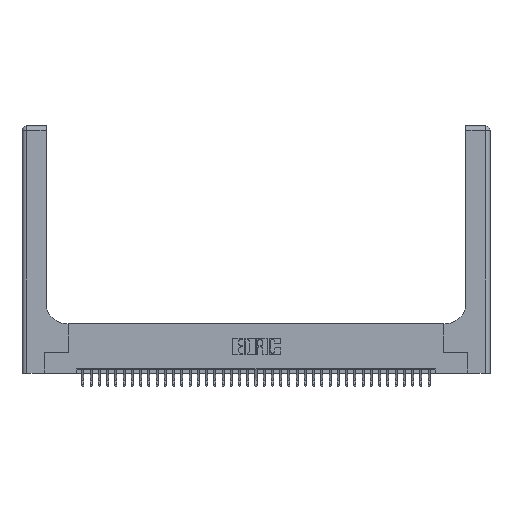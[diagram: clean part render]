
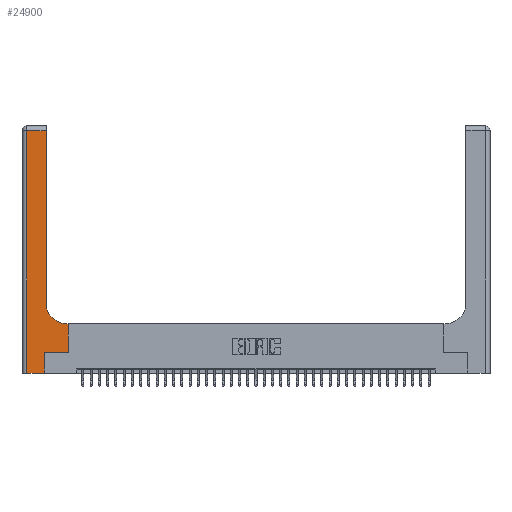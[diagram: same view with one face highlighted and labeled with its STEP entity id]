
A CAD part, top view. The second image highlights one B-rep face of the part: STEP entity #24900.
In plain terms, the highlighted planar face has unit normal (0, 0, 1).
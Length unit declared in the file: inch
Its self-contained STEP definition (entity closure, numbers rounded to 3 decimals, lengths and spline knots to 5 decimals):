
#95 = DIRECTION ( 'NONE',  ( 1., 0., 0. ) ) ;
#449 = VECTOR ( 'NONE', #18951, 39.37008 ) ;
#495 = EDGE_CURVE ( 'NONE', #4939, #36601, #34868, .T. ) ;
#773 = CARTESIAN_POINT ( 'NONE',  ( 0.2915, 0.6, 0.37 ) ) ;
#952 = LINE ( 'NONE', #773, #449 ) ;
#2243 = CARTESIAN_POINT ( 'NONE',  ( 0.5415, 0.6, 0.37 ) ) ;
#2503 = CARTESIAN_POINT ( 'NONE',  ( 0.06, 3., 0.37 ) ) ;
#2934 = VERTEX_POINT ( 'NONE', #2243 ) ;
#3071 = CARTESIAN_POINT ( 'NONE',  ( 0.5585, 0.25, 0.37 ) ) ;
#3129 = ORIENTED_EDGE ( 'NONE', *, *, #9283, .T. ) ;
#3180 = LINE ( 'NONE', #18246, #21992 ) ;
#4939 = VERTEX_POINT ( 'NONE', #29171 ) ;
#6209 = CARTESIAN_POINT ( 'NONE',  ( 0.06, 2.94, 0.37 ) ) ;
#6495 = ORIENTED_EDGE ( 'NONE', *, *, #19314, .T. ) ;
#7766 = DIRECTION ( 'NONE',  ( -1., 0., 0. ) ) ;
#8677 = PLANE ( 'NONE',  #22682 ) ;
#8778 = CARTESIAN_POINT ( 'NONE',  ( 0., 0., 0.37 ) ) ;
#9073 = ORIENTED_EDGE ( 'NONE', *, *, #16976, .T. ) ;
#9089 = CARTESIAN_POINT ( 'NONE',  ( 0., 3., 0.37 ) ) ;
#9207 = DIRECTION ( 'NONE',  ( 0., 1., 0. ) ) ;
#9229 = CARTESIAN_POINT ( 'NONE',  ( 0.06, 0., 0.37 ) ) ;
#9283 = EDGE_CURVE ( 'NONE', #36601, #21958, #17452, .T. ) ;
#9290 = EDGE_CURVE ( 'NONE', #37697, #36356, #27822, .T. ) ;
#9387 = LINE ( 'NONE', #2503, #24444 ) ;
#11012 = CARTESIAN_POINT ( 'NONE',  ( 0.5585, 0.25, 0.37 ) ) ;
#11868 = VECTOR ( 'NONE', #32856, 39.37008 ) ;
#12424 = ORIENTED_EDGE ( 'NONE', *, *, #9290, .T. ) ;
#13799 = CARTESIAN_POINT ( 'NONE',  ( 0., 2.94, 0.37 ) ) ;
#14481 = ORIENTED_EDGE ( 'NONE', *, *, #15938, .T. ) ;
#14742 = CARTESIAN_POINT ( 'NONE',  ( 0.5415, 0.85, 0.37 ) ) ;
#15938 = EDGE_CURVE ( 'NONE', #21958, #2934, #952, .T. ) ;
#16024 = VERTEX_POINT ( 'NONE', #6209 ) ;
#16976 = EDGE_CURVE ( 'NONE', #35573, #31599, #29206, .T. ) ;
#17452 = LINE ( 'NONE', #3071, #19821 ) ;
#17720 = CARTESIAN_POINT ( 'NONE',  ( 0.5585, 0.6, 0.37 ) ) ;
#18168 = VECTOR ( 'NONE', #7766, 39.37008 ) ;
#18206 = DIRECTION ( 'NONE',  ( 0., 1., 0. ) ) ;
#18246 = CARTESIAN_POINT ( 'NONE',  ( 0.269, 0., 0.37 ) ) ;
#18400 = DIRECTION ( 'NONE',  ( 1., 0., 0. ) ) ;
#18951 = DIRECTION ( 'NONE',  ( -1., 0., 0. ) ) ;
#19314 = EDGE_CURVE ( 'NONE', #31599, #16024, #34228, .T. ) ;
#19821 = VECTOR ( 'NONE', #18206, 39.37008 ) ;
#21958 = VERTEX_POINT ( 'NONE', #17720 ) ;
#21992 = VECTOR ( 'NONE', #9207, 39.37008 ) ;
#22091 = EDGE_CURVE ( 'NONE', #36356, #4939, #3180, .T. ) ;
#22132 = DIRECTION ( 'NONE',  ( 0., 1., 0. ) ) ;
#22682 = AXIS2_PLACEMENT_3D ( 'NONE', #9089, #29572, #32757 ) ;
#24063 = VECTOR ( 'NONE', #22132, 39.37008 ) ;
#24444 = VECTOR ( 'NONE', #34088, 39.37008 ) ;
#24900 = ADVANCED_FACE ( 'NONE', ( #31172 ), #8677, .F. ) ;
#25110 = ORIENTED_EDGE ( 'NONE', *, *, #35725, .T. ) ;
#26713 = DIRECTION ( 'NONE',  ( 0., 0., -1. ) ) ;
#27822 = LINE ( 'NONE', #8778, #11868 ) ;
#29027 = ORIENTED_EDGE ( 'NONE', *, *, #495, .T. ) ;
#29171 = CARTESIAN_POINT ( 'NONE',  ( 0.269, 0.25, 0.37 ) ) ;
#29206 = LINE ( 'NONE', #37038, #24063 ) ;
#29541 = CIRCLE ( 'NONE', #37992, 0.25 ) ;
#29572 = DIRECTION ( 'NONE',  ( 0., 0., -1. ) ) ;
#30585 = EDGE_LOOP ( 'NONE', ( #9073, #6495, #25110, #12424, #35002, #29027, #3129, #14481, #30800 ) ) ;
#30800 = ORIENTED_EDGE ( 'NONE', *, *, #36248, .T. ) ;
#31172 = FACE_OUTER_BOUND ( 'NONE', #30585, .T. ) ;
#31599 = VERTEX_POINT ( 'NONE', #34685 ) ;
#31879 = CARTESIAN_POINT ( 'NONE',  ( 0.2915, 0.85, 0.37 ) ) ;
#32757 = DIRECTION ( 'NONE',  ( -1., 0., 0. ) ) ;
#32856 = DIRECTION ( 'NONE',  ( 1., 0., 0. ) ) ;
#33786 = CARTESIAN_POINT ( 'NONE',  ( 0.269, 0., 0.37 ) ) ;
#34088 = DIRECTION ( 'NONE',  ( 0., -1., 0. ) ) ;
#34228 = LINE ( 'NONE', #13799, #18168 ) ;
#34685 = CARTESIAN_POINT ( 'NONE',  ( 0.2915, 2.94, 0.37 ) ) ;
#34868 = LINE ( 'NONE', #38985, #35339 ) ;
#35002 = ORIENTED_EDGE ( 'NONE', *, *, #22091, .T. ) ;
#35339 = VECTOR ( 'NONE', #18400, 39.37008 ) ;
#35573 = VERTEX_POINT ( 'NONE', #31879 ) ;
#35725 = EDGE_CURVE ( 'NONE', #16024, #37697, #9387, .T. ) ;
#36248 = EDGE_CURVE ( 'NONE', #2934, #35573, #29541, .T. ) ;
#36356 = VERTEX_POINT ( 'NONE', #33786 ) ;
#36601 = VERTEX_POINT ( 'NONE', #11012 ) ;
#37038 = CARTESIAN_POINT ( 'NONE',  ( 0.2915, 3., 0.37 ) ) ;
#37697 = VERTEX_POINT ( 'NONE', #9229 ) ;
#37992 = AXIS2_PLACEMENT_3D ( 'NONE', #14742, #26713, #95 ) ;
#38985 = CARTESIAN_POINT ( 'NONE',  ( 0.269, 0.25, 0.37 ) ) ;
